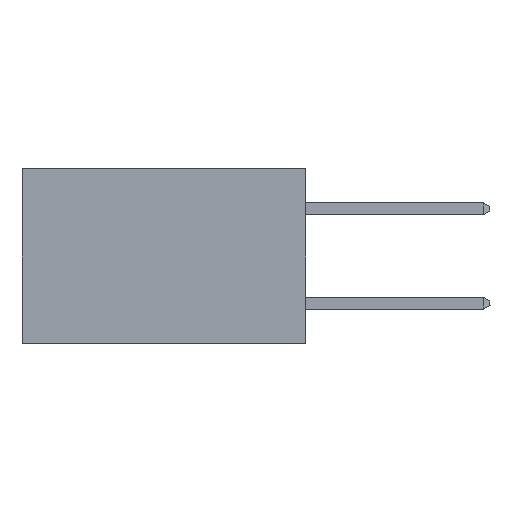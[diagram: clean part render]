
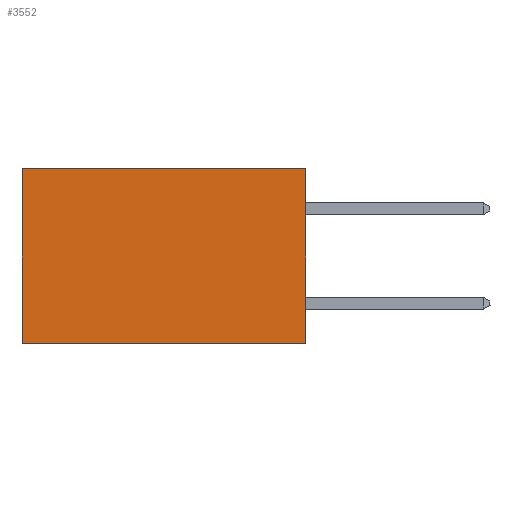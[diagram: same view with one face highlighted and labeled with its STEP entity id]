
A CAD part, left-side view. The second image highlights one B-rep face of the part: STEP entity #3552.
In plain terms, the highlighted planar face has unit normal (-1, 0, 0).
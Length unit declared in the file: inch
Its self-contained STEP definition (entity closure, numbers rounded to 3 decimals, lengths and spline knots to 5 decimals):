
#634 = CARTESIAN_POINT ( 'NONE',  ( 0.2615, 0., -0.37 ) ) ;
#845 = PLANE ( 'NONE',  #6369 ) ;
#1274 = VERTEX_POINT ( 'NONE', #15639 ) ;
#1354 = DIRECTION ( 'NONE',  ( 0., 0., -1. ) ) ;
#1717 = DIRECTION ( 'NONE',  ( 1., 0., 0. ) ) ;
#2478 = CARTESIAN_POINT ( 'NONE',  ( 0.2615, 0., -0.37 ) ) ;
#2773 = FACE_OUTER_BOUND ( 'NONE', #13494, .T. ) ;
#3061 = ORIENTED_EDGE ( 'NONE', *, *, #26872, .F. ) ;
#3552 = ADVANCED_FACE ( 'NONE', ( #2773 ), #845, .F. ) ;
#3905 = CARTESIAN_POINT ( 'NONE',  ( 0.2615, 0., -0.37 ) ) ;
#4141 = LINE ( 'NONE', #7468, #15467 ) ;
#4406 = DIRECTION ( 'NONE',  ( 0., 1., 0. ) ) ;
#4441 = ORIENTED_EDGE ( 'NONE', *, *, #5078, .T. ) ;
#4915 = VERTEX_POINT ( 'NONE', #2478 ) ;
#5078 = EDGE_CURVE ( 'NONE', #7625, #6152, #17025, .T. ) ;
#5296 = EDGE_CURVE ( 'NONE', #4915, #1274, #21618, .T. ) ;
#6152 = VERTEX_POINT ( 'NONE', #8987 ) ;
#6369 = AXIS2_PLACEMENT_3D ( 'NONE', #634, #1717, #1354 ) ;
#7468 = CARTESIAN_POINT ( 'NONE',  ( 0.2615, 0.6, -0.37 ) ) ;
#7625 = VERTEX_POINT ( 'NONE', #21058 ) ;
#8987 = CARTESIAN_POINT ( 'NONE',  ( 0.2615, 0.6, 0. ) ) ;
#9488 = VECTOR ( 'NONE', #23649, 39.37008 ) ;
#10427 = VECTOR ( 'NONE', #4406, 39.37008 ) ;
#12655 = ORIENTED_EDGE ( 'NONE', *, *, #5296, .F. ) ;
#13494 = EDGE_LOOP ( 'NONE', ( #21792, #12655, #3061, #4441 ) ) ;
#15052 = VECTOR ( 'NONE', #20952, 39.37008 ) ;
#15309 = CARTESIAN_POINT ( 'NONE',  ( 0.2615, 0., -0.37 ) ) ;
#15467 = VECTOR ( 'NONE', #24281, 39.37008 ) ;
#15639 = CARTESIAN_POINT ( 'NONE',  ( 0.2615, 0.6, -0.37 ) ) ;
#17025 = LINE ( 'NONE', #20955, #15052 ) ;
#20952 = DIRECTION ( 'NONE',  ( 0., 1., 0. ) ) ;
#20955 = CARTESIAN_POINT ( 'NONE',  ( 0.2615, 0., 0. ) ) ;
#21058 = CARTESIAN_POINT ( 'NONE',  ( 0.2615, 0., 0. ) ) ;
#21618 = LINE ( 'NONE', #3905, #10427 ) ;
#21792 = ORIENTED_EDGE ( 'NONE', *, *, #25093, .T. ) ;
#23649 = DIRECTION ( 'NONE',  ( 0., 0., -1. ) ) ;
#24281 = DIRECTION ( 'NONE',  ( 0., 0., -1. ) ) ;
#25093 = EDGE_CURVE ( 'NONE', #6152, #1274, #4141, .T. ) ;
#25546 = LINE ( 'NONE', #15309, #9488 ) ;
#26872 = EDGE_CURVE ( 'NONE', #7625, #4915, #25546, .T. ) ;
